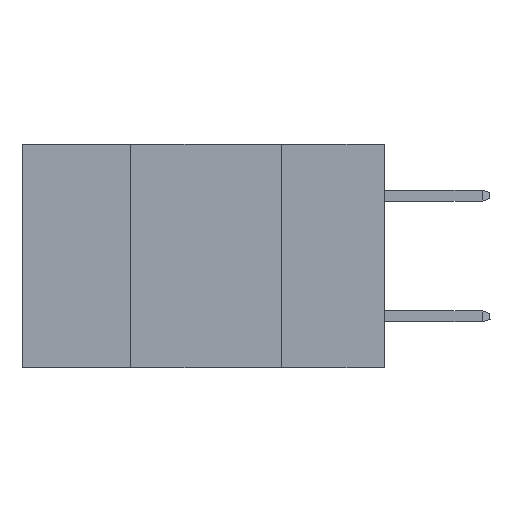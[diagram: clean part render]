
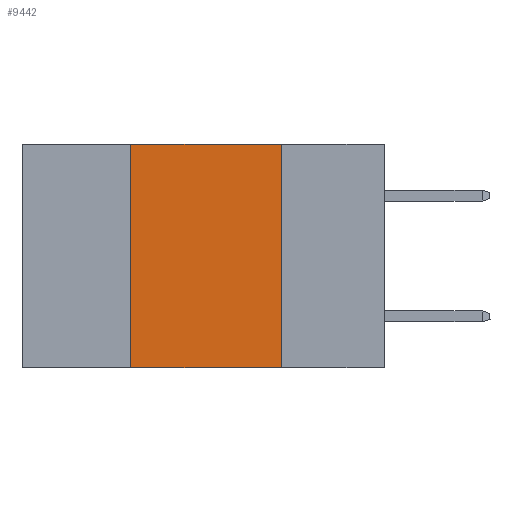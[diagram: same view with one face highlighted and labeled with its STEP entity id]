
A CAD part, left-side view. The second image highlights one B-rep face of the part: STEP entity #9442.
In plain terms, the highlighted planar face has unit normal (-1, 0, 0).
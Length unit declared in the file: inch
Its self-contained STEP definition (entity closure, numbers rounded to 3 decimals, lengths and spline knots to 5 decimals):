
#181 = EDGE_LOOP ( 'NONE', ( #2678, #2715, #2867, #1362 ) ) ;
#759 = VERTEX_POINT ( 'NONE', #8675 ) ;
#1362 = ORIENTED_EDGE ( 'NONE', *, *, #1979, .T. ) ;
#1707 = VECTOR ( 'NONE', #16003, 39.37008 ) ;
#1979 = EDGE_CURVE ( 'NONE', #759, #15899, #16497, .T. ) ;
#2678 = ORIENTED_EDGE ( 'NONE', *, *, #7144, .F. ) ;
#2715 = ORIENTED_EDGE ( 'NONE', *, *, #6106, .F. ) ;
#2867 = ORIENTED_EDGE ( 'NONE', *, *, #3012, .F. ) ;
#3012 = EDGE_CURVE ( 'NONE', #759, #3975, #18599, .T. ) ;
#3046 = CARTESIAN_POINT ( 'NONE',  ( 0., 0.42, -0.37 ) ) ;
#3491 = VECTOR ( 'NONE', #12121, 39.37008 ) ;
#3849 = DIRECTION ( 'NONE',  ( 0., 0., -1. ) ) ;
#3879 = DIRECTION ( 'NONE',  ( 1., 0., 0. ) ) ;
#3923 = CARTESIAN_POINT ( 'NONE',  ( 0., 0.6, 0. ) ) ;
#3926 = PLANE ( 'NONE',  #17102 ) ;
#3975 = VERTEX_POINT ( 'NONE', #4664 ) ;
#4213 = CARTESIAN_POINT ( 'NONE',  ( 0., 0.6, -0.37 ) ) ;
#4609 = DIRECTION ( 'NONE',  ( 0., 0., 1. ) ) ;
#4664 = CARTESIAN_POINT ( 'NONE',  ( 0., 0.42, 0. ) ) ;
#6106 = EDGE_CURVE ( 'NONE', #3975, #16306, #15225, .T. ) ;
#7144 = EDGE_CURVE ( 'NONE', #16306, #15899, #10084, .T. ) ;
#8675 = CARTESIAN_POINT ( 'NONE',  ( 0., 0.42, -0.37 ) ) ;
#9266 = CARTESIAN_POINT ( 'NONE',  ( 0., 0.17, -0.37 ) ) ;
#9327 = DIRECTION ( 'NONE',  ( 0., 0., -1. ) ) ;
#9442 = ADVANCED_FACE ( 'NONE', ( #15334 ), #3926, .F. ) ;
#10084 = LINE ( 'NONE', #9266, #13444 ) ;
#11282 = CARTESIAN_POINT ( 'NONE',  ( 0., 0.17, 0. ) ) ;
#11598 = VECTOR ( 'NONE', #4609, 39.37008 ) ;
#12121 = DIRECTION ( 'NONE',  ( 0., -1., 0. ) ) ;
#12920 = CARTESIAN_POINT ( 'NONE',  ( 0., 0.6, 0. ) ) ;
#13444 = VECTOR ( 'NONE', #9327, 39.37008 ) ;
#15225 = LINE ( 'NONE', #12920, #3491 ) ;
#15334 = FACE_OUTER_BOUND ( 'NONE', #181, .T. ) ;
#15899 = VERTEX_POINT ( 'NONE', #18054 ) ;
#16003 = DIRECTION ( 'NONE',  ( 0., -1., 0. ) ) ;
#16306 = VERTEX_POINT ( 'NONE', #11282 ) ;
#16497 = LINE ( 'NONE', #4213, #1707 ) ;
#17102 = AXIS2_PLACEMENT_3D ( 'NONE', #3923, #3879, #3849 ) ;
#18054 = CARTESIAN_POINT ( 'NONE',  ( 0., 0.17, -0.37 ) ) ;
#18599 = LINE ( 'NONE', #3046, #11598 ) ;
